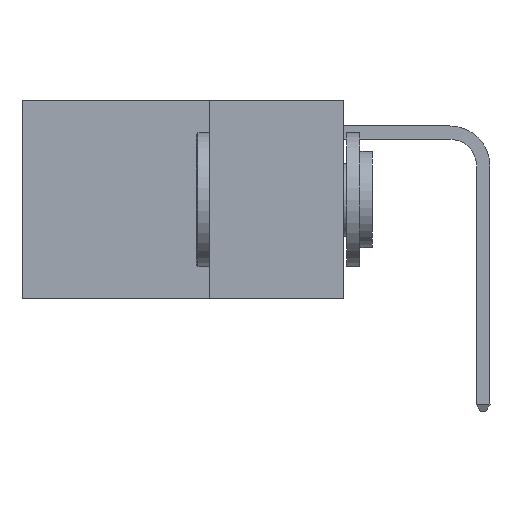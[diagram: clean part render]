
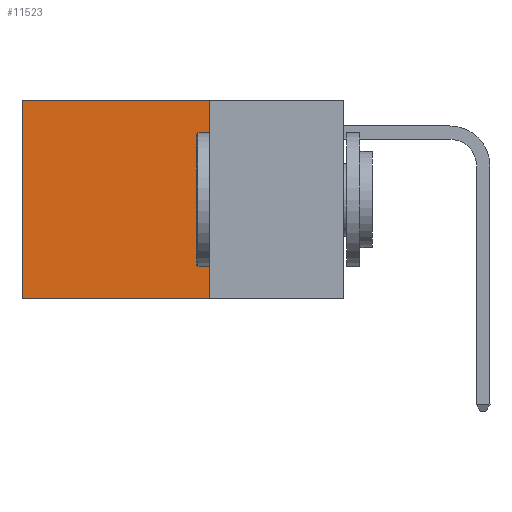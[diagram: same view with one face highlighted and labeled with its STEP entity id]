
A CAD part, left-side view. The second image highlights one B-rep face of the part: STEP entity #11523.
In plain terms, the highlighted planar face has unit normal (-1, 0, 0).
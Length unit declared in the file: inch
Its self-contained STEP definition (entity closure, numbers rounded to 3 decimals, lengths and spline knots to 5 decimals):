
#337 = EDGE_CURVE ( 'NONE', #12837, #19252, #13052, .T. ) ;
#661 = CARTESIAN_POINT ( 'NONE',  ( 0.2625, 0.25, -0.37 ) ) ;
#1149 = VECTOR ( 'NONE', #17529, 39.37008 ) ;
#1336 = CARTESIAN_POINT ( 'NONE',  ( 0.2625, 0.6, 0. ) ) ;
#1708 = EDGE_CURVE ( 'NONE', #12837, #17322, #16143, .T. ) ;
#2007 = ORIENTED_EDGE ( 'NONE', *, *, #3599, .T. ) ;
#3599 = EDGE_CURVE ( 'NONE', #19252, #10188, #17896, .T. ) ;
#3663 = CARTESIAN_POINT ( 'NONE',  ( 0.2625, 0.25, -0.37 ) ) ;
#3837 = VECTOR ( 'NONE', #12113, 39.37008 ) ;
#3914 = CARTESIAN_POINT ( 'NONE',  ( 0.2625, 0.25, 0. ) ) ;
#4252 = ORIENTED_EDGE ( 'NONE', *, *, #1708, .F. ) ;
#5090 = EDGE_CURVE ( 'NONE', #17322, #10188, #7927, .T. ) ;
#5134 = DIRECTION ( 'NONE',  ( 0., 1., 0. ) ) ;
#5236 = CARTESIAN_POINT ( 'NONE',  ( 0.2625, 0.25, 0. ) ) ;
#6587 = ORIENTED_EDGE ( 'NONE', *, *, #337, .T. ) ;
#7620 = CARTESIAN_POINT ( 'NONE',  ( 0.2625, 0.6, 0. ) ) ;
#7927 = LINE ( 'NONE', #3663, #9537 ) ;
#8879 = CARTESIAN_POINT ( 'NONE',  ( 0.2625, 0.25, 0. ) ) ;
#8932 = EDGE_LOOP ( 'NONE', ( #2007, #17416, #4252, #6587 ) ) ;
#9537 = VECTOR ( 'NONE', #5134, 39.37008 ) ;
#9662 = DIRECTION ( 'NONE',  ( 0., 0., -1. ) ) ;
#10188 = VERTEX_POINT ( 'NONE', #10532 ) ;
#10365 = AXIS2_PLACEMENT_3D ( 'NONE', #5236, #15715, #9662 ) ;
#10532 = CARTESIAN_POINT ( 'NONE',  ( 0.2625, 0.6, -0.37 ) ) ;
#11523 = ADVANCED_FACE ( 'NONE', ( #18396 ), #17191, .F. ) ;
#11645 = CARTESIAN_POINT ( 'NONE',  ( 0.2625, 0.25, 0. ) ) ;
#12113 = DIRECTION ( 'NONE',  ( 0., 0., -1. ) ) ;
#12837 = VERTEX_POINT ( 'NONE', #8879 ) ;
#12940 = DIRECTION ( 'NONE',  ( 0., 0., -1. ) ) ;
#13052 = LINE ( 'NONE', #3914, #1149 ) ;
#15715 = DIRECTION ( 'NONE',  ( 1., 0., 0. ) ) ;
#16143 = LINE ( 'NONE', #11645, #18568 ) ;
#17191 = PLANE ( 'NONE',  #10365 ) ;
#17322 = VERTEX_POINT ( 'NONE', #661 ) ;
#17416 = ORIENTED_EDGE ( 'NONE', *, *, #5090, .F. ) ;
#17529 = DIRECTION ( 'NONE',  ( 0., 1., 0. ) ) ;
#17896 = LINE ( 'NONE', #7620, #3837 ) ;
#18396 = FACE_OUTER_BOUND ( 'NONE', #8932, .T. ) ;
#18568 = VECTOR ( 'NONE', #12940, 39.37008 ) ;
#19252 = VERTEX_POINT ( 'NONE', #1336 ) ;
